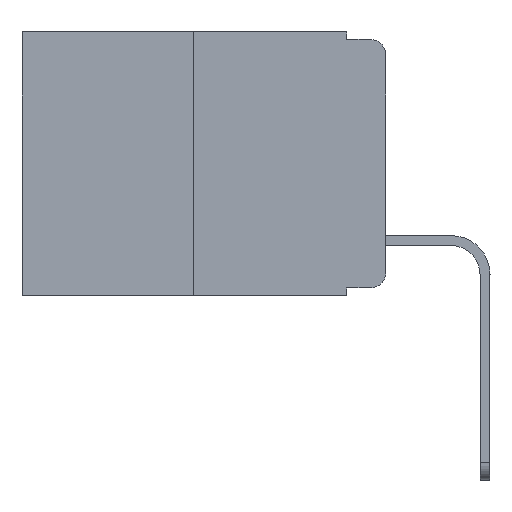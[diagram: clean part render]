
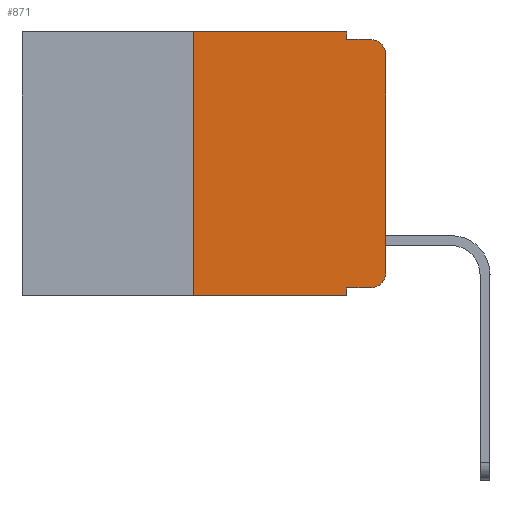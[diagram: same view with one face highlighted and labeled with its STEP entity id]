
A CAD part, left-side view. The second image highlights one B-rep face of the part: STEP entity #871.
In plain terms, the highlighted planar face has unit normal (-1, 0, 0).
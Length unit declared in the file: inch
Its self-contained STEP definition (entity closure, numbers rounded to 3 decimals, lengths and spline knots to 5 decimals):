
#227 = ORIENTED_EDGE ( 'NONE', *, *, #11126, .F. ) ;
#502 = DIRECTION ( 'NONE',  ( 0., 0., 1. ) ) ;
#780 = EDGE_CURVE ( 'NONE', #8361, #10329, #8030, .T. ) ;
#871 = ADVANCED_FACE ( 'NONE', ( #3812 ), #6545, .F. ) ;
#951 = VERTEX_POINT ( 'NONE', #5216 ) ;
#1068 = EDGE_CURVE ( 'NONE', #8170, #8345, #6711, .T. ) ;
#1318 = CARTESIAN_POINT ( 'NONE',  ( 0., 0.02, -0.01 ) ) ;
#1614 = DIRECTION ( 'NONE',  ( 0., -1., 0. ) ) ;
#1988 = VERTEX_POINT ( 'NONE', #2922 ) ;
#2435 = EDGE_LOOP ( 'NONE', ( #3488, #9165, #10760, #13347, #7780, #227, #6479, #3476, #6678, #12957 ) ) ;
#2922 = CARTESIAN_POINT ( 'NONE',  ( 0., 0.051, -0.01 ) ) ;
#2928 = CARTESIAN_POINT ( 'NONE',  ( 0., 0., 0. ) ) ;
#3050 = VECTOR ( 'NONE', #1614, 39.37008 ) ;
#3213 = CARTESIAN_POINT ( 'NONE',  ( 0., 0.051, -0.343 ) ) ;
#3220 = AXIS2_PLACEMENT_3D ( 'NONE', #11268, #13541, #6597 ) ;
#3418 = DIRECTION ( 'NONE',  ( 0., 0., -1. ) ) ;
#3476 = ORIENTED_EDGE ( 'NONE', *, *, #1068, .F. ) ;
#3488 = ORIENTED_EDGE ( 'NONE', *, *, #11600, .T. ) ;
#3692 = VERTEX_POINT ( 'NONE', #1318 ) ;
#3812 = FACE_OUTER_BOUND ( 'NONE', #2435, .T. ) ;
#4311 = CARTESIAN_POINT ( 'NONE',  ( 0., 0.02, -0.333 ) ) ;
#4457 = CARTESIAN_POINT ( 'NONE',  ( 0., 0., -0.313 ) ) ;
#4540 = CARTESIAN_POINT ( 'NONE',  ( 0., 0.02, -0.313 ) ) ;
#4623 = VECTOR ( 'NONE', #13996, 39.37008 ) ;
#4678 = VERTEX_POINT ( 'NONE', #11416 ) ;
#4919 = EDGE_CURVE ( 'NONE', #7425, #8372, #12230, .T. ) ;
#5108 = AXIS2_PLACEMENT_3D ( 'NONE', #4540, #10478, #3418 ) ;
#5216 = CARTESIAN_POINT ( 'NONE',  ( 0., 0., -0.03 ) ) ;
#5380 = CARTESIAN_POINT ( 'NONE',  ( 0., 0.051, 0. ) ) ;
#5580 = CARTESIAN_POINT ( 'NONE',  ( 0., 0.051, -0.333 ) ) ;
#6426 = EDGE_CURVE ( 'NONE', #10329, #1988, #8658, .T. ) ;
#6479 = ORIENTED_EDGE ( 'NONE', *, *, #9924, .T. ) ;
#6545 = PLANE ( 'NONE',  #3220 ) ;
#6597 = DIRECTION ( 'NONE',  ( 0., 0., -1. ) ) ;
#6678 = ORIENTED_EDGE ( 'NONE', *, *, #13371, .T. ) ;
#6711 = LINE ( 'NONE', #9609, #7642 ) ;
#7048 = CARTESIAN_POINT ( 'NONE',  ( 0., 0.051, 0. ) ) ;
#7123 = CARTESIAN_POINT ( 'NONE',  ( 0., 0.02, -0.03 ) ) ;
#7146 = DIRECTION ( 'NONE',  ( 0., 0., -1. ) ) ;
#7399 = CARTESIAN_POINT ( 'NONE',  ( 0., 0.051, -0.01 ) ) ;
#7425 = VERTEX_POINT ( 'NONE', #4311 ) ;
#7473 = LINE ( 'NONE', #12867, #14637 ) ;
#7642 = VECTOR ( 'NONE', #14958, 39.37008 ) ;
#7780 = ORIENTED_EDGE ( 'NONE', *, *, #780, .F. ) ;
#8030 = LINE ( 'NONE', #10865, #8963 ) ;
#8047 = CARTESIAN_POINT ( 'NONE',  ( 0., 0.25, 0. ) ) ;
#8137 = LINE ( 'NONE', #5580, #4623 ) ;
#8170 = VERTEX_POINT ( 'NONE', #10138 ) ;
#8208 = DIRECTION ( 'NONE',  ( 0., -1., 0. ) ) ;
#8217 = LINE ( 'NONE', #8311, #8958 ) ;
#8311 = CARTESIAN_POINT ( 'NONE',  ( 0., 0.473, -0.343 ) ) ;
#8345 = VERTEX_POINT ( 'NONE', #3213 ) ;
#8361 = VERTEX_POINT ( 'NONE', #8047 ) ;
#8372 = VERTEX_POINT ( 'NONE', #4457 ) ;
#8658 = LINE ( 'NONE', #7048, #9046 ) ;
#8958 = VECTOR ( 'NONE', #8208, 39.37008 ) ;
#8963 = VECTOR ( 'NONE', #14551, 39.37008 ) ;
#9046 = VECTOR ( 'NONE', #7146, 39.37008 ) ;
#9165 = ORIENTED_EDGE ( 'NONE', *, *, #13374, .T. ) ;
#9335 = EDGE_CURVE ( 'NONE', #1988, #3692, #14831, .T. ) ;
#9609 = CARTESIAN_POINT ( 'NONE',  ( 0., 0.051, 0. ) ) ;
#9924 = EDGE_CURVE ( 'NONE', #4678, #8345, #8217, .T. ) ;
#9971 = AXIS2_PLACEMENT_3D ( 'NONE', #7123, #15269, #14296 ) ;
#10138 = CARTESIAN_POINT ( 'NONE',  ( 0., 0.051, -0.333 ) ) ;
#10329 = VERTEX_POINT ( 'NONE', #5380 ) ;
#10478 = DIRECTION ( 'NONE',  ( -1., 0., 0. ) ) ;
#10760 = ORIENTED_EDGE ( 'NONE', *, *, #9335, .F. ) ;
#10865 = CARTESIAN_POINT ( 'NONE',  ( 0., 0.473, 0. ) ) ;
#11126 = EDGE_CURVE ( 'NONE', #4678, #8361, #7473, .T. ) ;
#11268 = CARTESIAN_POINT ( 'NONE',  ( 0., 0.473, 0. ) ) ;
#11416 = CARTESIAN_POINT ( 'NONE',  ( 0., 0.25, -0.343 ) ) ;
#11522 = VECTOR ( 'NONE', #502, 39.37008 ) ;
#11600 = EDGE_CURVE ( 'NONE', #8372, #951, #13171, .T. ) ;
#12230 = CIRCLE ( 'NONE', #5108, 0.02 ) ;
#12867 = CARTESIAN_POINT ( 'NONE',  ( 0., 0.25, 0. ) ) ;
#12957 = ORIENTED_EDGE ( 'NONE', *, *, #4919, .T. ) ;
#13171 = LINE ( 'NONE', #2928, #11522 ) ;
#13309 = CIRCLE ( 'NONE', #9971, 0.02 ) ;
#13347 = ORIENTED_EDGE ( 'NONE', *, *, #6426, .F. ) ;
#13371 = EDGE_CURVE ( 'NONE', #8170, #7425, #8137, .T. ) ;
#13374 = EDGE_CURVE ( 'NONE', #951, #3692, #13309, .T. ) ;
#13541 = DIRECTION ( 'NONE',  ( 1., 0., 0. ) ) ;
#13996 = DIRECTION ( 'NONE',  ( 0., -1., 0. ) ) ;
#14296 = DIRECTION ( 'NONE',  ( 0., 0., -1. ) ) ;
#14551 = DIRECTION ( 'NONE',  ( 0., -1., 0. ) ) ;
#14637 = VECTOR ( 'NONE', #14994, 39.37008 ) ;
#14831 = LINE ( 'NONE', #7399, #3050 ) ;
#14958 = DIRECTION ( 'NONE',  ( 0., 0., -1. ) ) ;
#14994 = DIRECTION ( 'NONE',  ( 0., 0., 1. ) ) ;
#15269 = DIRECTION ( 'NONE',  ( -1., 0., 0. ) ) ;
